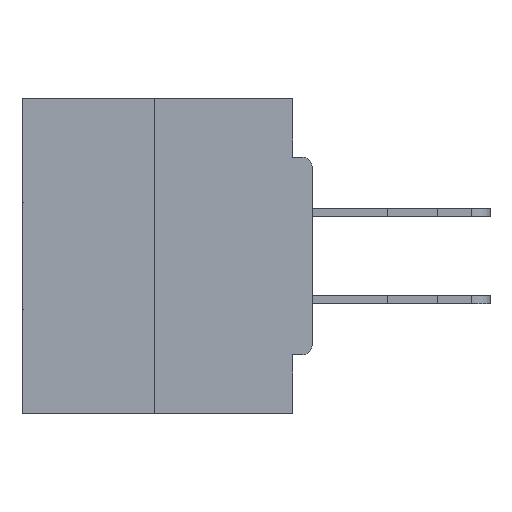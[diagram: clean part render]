
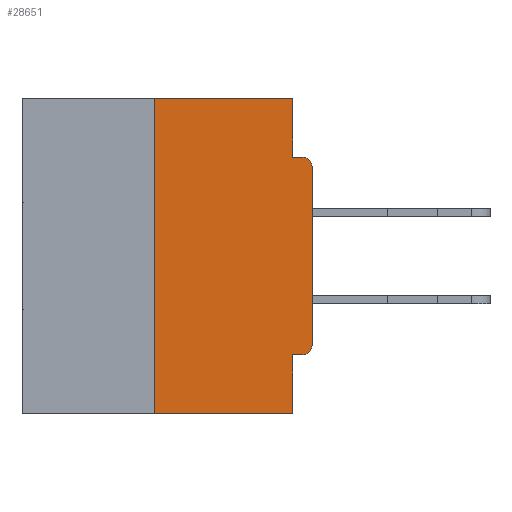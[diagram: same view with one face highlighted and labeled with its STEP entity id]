
A CAD part, left-side view. The second image highlights one B-rep face of the part: STEP entity #28651.
In plain terms, the highlighted planar face has unit normal (-1, 0, 0).
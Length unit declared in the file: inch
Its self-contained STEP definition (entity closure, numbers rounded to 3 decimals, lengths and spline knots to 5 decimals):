
#411 = VECTOR ( 'NONE', #34807, 39.37008 ) ;
#671 = AXIS2_PLACEMENT_3D ( 'NONE', #11675, #22287, #5301 ) ;
#706 = EDGE_CURVE ( 'NONE', #16533, #18559, #27169, .T. ) ;
#1371 = ORIENTED_EDGE ( 'NONE', *, *, #20525, .T. ) ;
#2008 = DIRECTION ( 'NONE',  ( 0., -1., 0. ) ) ;
#2135 = CARTESIAN_POINT ( 'NONE',  ( 0., 0.031, 0. ) ) ;
#2930 = CARTESIAN_POINT ( 'NONE',  ( 0., 0.031, 0. ) ) ;
#2970 = DIRECTION ( 'NONE',  ( 0., 0., -1. ) ) ;
#3208 = CARTESIAN_POINT ( 'NONE',  ( 0., 0.015, -0.0935 ) ) ;
#4015 = CARTESIAN_POINT ( 'NONE',  ( 0., 0.25, -0.5 ) ) ;
#4180 = DIRECTION ( 'NONE',  ( 0., 0., -1. ) ) ;
#4182 = LINE ( 'NONE', #30579, #6044 ) ;
#4464 = VECTOR ( 'NONE', #12394, 39.37008 ) ;
#5301 = DIRECTION ( 'NONE',  ( 0., 0., -1. ) ) ;
#6044 = VECTOR ( 'NONE', #4180, 39.37008 ) ;
#6209 = CARTESIAN_POINT ( 'NONE',  ( 0., 0., -0.4065 ) ) ;
#6724 = VERTEX_POINT ( 'NONE', #11844 ) ;
#7452 = CIRCLE ( 'NONE', #671, 0.015 ) ;
#7489 = CARTESIAN_POINT ( 'NONE',  ( 0., 0.46, -0.5 ) ) ;
#7887 = CARTESIAN_POINT ( 'NONE',  ( 0., 0., -0.1085 ) ) ;
#8907 = EDGE_LOOP ( 'NONE', ( #11137, #22086, #26587, #15065, #19484, #31266, #1371, #20864, #15655, #26155 ) ) ;
#9447 = EDGE_CURVE ( 'NONE', #18559, #23635, #29849, .T. ) ;
#11119 = EDGE_CURVE ( 'NONE', #12372, #29083, #7452, .T. ) ;
#11137 = ORIENTED_EDGE ( 'NONE', *, *, #706, .F. ) ;
#11236 = LINE ( 'NONE', #6209, #32847 ) ;
#11293 = CARTESIAN_POINT ( 'NONE',  ( 0., 0.46, 0. ) ) ;
#11306 = CARTESIAN_POINT ( 'NONE',  ( 0., 0.031, -0.0935 ) ) ;
#11401 = LINE ( 'NONE', #32540, #4464 ) ;
#11675 = CARTESIAN_POINT ( 'NONE',  ( 0., 0.015, -0.1085 ) ) ;
#11844 = CARTESIAN_POINT ( 'NONE',  ( 0., 0.031, -0.4065 ) ) ;
#12172 = DIRECTION ( 'NONE',  ( 0., -1., 0. ) ) ;
#12372 = VERTEX_POINT ( 'NONE', #7887 ) ;
#12394 = DIRECTION ( 'NONE',  ( 0., 0., 1. ) ) ;
#12403 = CARTESIAN_POINT ( 'NONE',  ( 0., 0.015, -0.4065 ) ) ;
#12490 = EDGE_CURVE ( 'NONE', #13862, #29610, #20968, .T. ) ;
#13469 = AXIS2_PLACEMENT_3D ( 'NONE', #32214, #17044, #20118 ) ;
#13862 = VERTEX_POINT ( 'NONE', #4015 ) ;
#14024 = DIRECTION ( 'NONE',  ( 0., 0., 1. ) ) ;
#14049 = EDGE_CURVE ( 'NONE', #14817, #6724, #11236, .T. ) ;
#14509 = VERTEX_POINT ( 'NONE', #23379 ) ;
#14817 = VERTEX_POINT ( 'NONE', #12403 ) ;
#15065 = ORIENTED_EDGE ( 'NONE', *, *, #15281, .F. ) ;
#15281 = EDGE_CURVE ( 'NONE', #6724, #29610, #4182, .T. ) ;
#15655 = ORIENTED_EDGE ( 'NONE', *, *, #19425, .F. ) ;
#16381 = VECTOR ( 'NONE', #14024, 39.37008 ) ;
#16533 = VERTEX_POINT ( 'NONE', #24349 ) ;
#17044 = DIRECTION ( 'NONE',  ( 1., 0., 0. ) ) ;
#18559 = VERTEX_POINT ( 'NONE', #2135 ) ;
#19425 = EDGE_CURVE ( 'NONE', #23635, #29083, #34948, .T. ) ;
#19484 = ORIENTED_EDGE ( 'NONE', *, *, #14049, .F. ) ;
#20118 = DIRECTION ( 'NONE',  ( 0., 0., -1. ) ) ;
#20525 = EDGE_CURVE ( 'NONE', #14509, #12372, #11401, .T. ) ;
#20855 = CARTESIAN_POINT ( 'NONE',  ( 0., 0., -0.0935 ) ) ;
#20864 = ORIENTED_EDGE ( 'NONE', *, *, #11119, .T. ) ;
#20968 = LINE ( 'NONE', #7489, #26972 ) ;
#21389 = EDGE_CURVE ( 'NONE', #13862, #16533, #24222, .T. ) ;
#22086 = ORIENTED_EDGE ( 'NONE', *, *, #21389, .F. ) ;
#22287 = DIRECTION ( 'NONE',  ( -1., 0., 0. ) ) ;
#23379 = CARTESIAN_POINT ( 'NONE',  ( 0., 0., -0.3915 ) ) ;
#23635 = VERTEX_POINT ( 'NONE', #11306 ) ;
#23654 = DIRECTION ( 'NONE',  ( 0., 0., -1. ) ) ;
#23958 = DIRECTION ( 'NONE',  ( -1., 0., 0. ) ) ;
#24222 = LINE ( 'NONE', #26235, #16381 ) ;
#24349 = CARTESIAN_POINT ( 'NONE',  ( 0., 0.25, 0. ) ) ;
#25510 = CARTESIAN_POINT ( 'NONE',  ( 0., 0.031, -0.5 ) ) ;
#26155 = ORIENTED_EDGE ( 'NONE', *, *, #9447, .F. ) ;
#26178 = PLANE ( 'NONE',  #13469 ) ;
#26235 = CARTESIAN_POINT ( 'NONE',  ( 0., 0.25, 0. ) ) ;
#26587 = ORIENTED_EDGE ( 'NONE', *, *, #12490, .T. ) ;
#26972 = VECTOR ( 'NONE', #2008, 39.37008 ) ;
#27126 = VECTOR ( 'NONE', #12172, 39.37008 ) ;
#27169 = LINE ( 'NONE', #11293, #411 ) ;
#28651 = ADVANCED_FACE ( 'NONE', ( #37510 ), #26178, .F. ) ;
#29083 = VERTEX_POINT ( 'NONE', #3208 ) ;
#29495 = CARTESIAN_POINT ( 'NONE',  ( 0., 0.015, -0.3915 ) ) ;
#29610 = VERTEX_POINT ( 'NONE', #25510 ) ;
#29849 = LINE ( 'NONE', #2930, #35844 ) ;
#30579 = CARTESIAN_POINT ( 'NONE',  ( 0., 0.031, -0.5 ) ) ;
#31175 = EDGE_CURVE ( 'NONE', #14817, #14509, #36367, .T. ) ;
#31266 = ORIENTED_EDGE ( 'NONE', *, *, #31175, .T. ) ;
#32214 = CARTESIAN_POINT ( 'NONE',  ( 0., 0.46, 0. ) ) ;
#32540 = CARTESIAN_POINT ( 'NONE',  ( 0., 0., 0. ) ) ;
#32847 = VECTOR ( 'NONE', #35272, 39.37008 ) ;
#34807 = DIRECTION ( 'NONE',  ( 0., -1., 0. ) ) ;
#34948 = LINE ( 'NONE', #20855, #27126 ) ;
#35272 = DIRECTION ( 'NONE',  ( 0., 1., 0. ) ) ;
#35844 = VECTOR ( 'NONE', #23654, 39.37008 ) ;
#35984 = AXIS2_PLACEMENT_3D ( 'NONE', #29495, #23958, #2970 ) ;
#36367 = CIRCLE ( 'NONE', #35984, 0.015 ) ;
#37510 = FACE_OUTER_BOUND ( 'NONE', #8907, .T. ) ;
